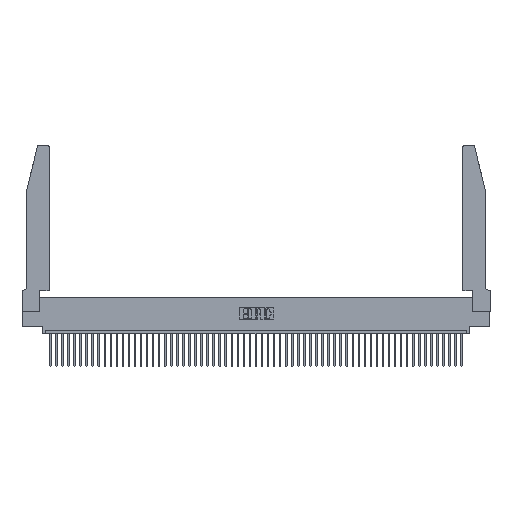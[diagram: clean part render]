
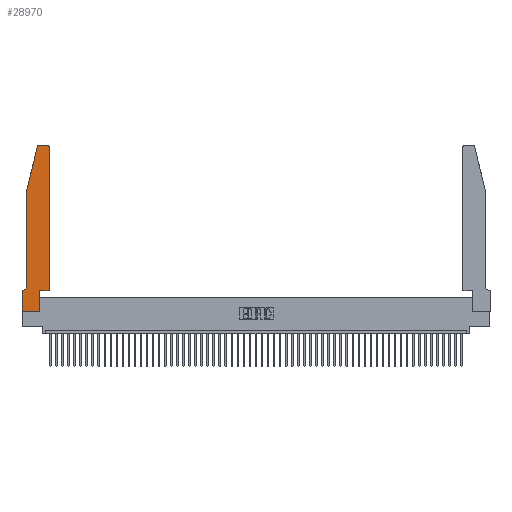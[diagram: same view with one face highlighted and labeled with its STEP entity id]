
A CAD part, top view. The second image highlights one B-rep face of the part: STEP entity #28970.
In plain terms, the highlighted planar face has unit normal (0, 0, 1).
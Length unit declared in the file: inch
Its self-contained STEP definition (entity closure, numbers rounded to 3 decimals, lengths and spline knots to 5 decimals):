
#1475 = DIRECTION ( 'NONE',  ( 1., 0., 0. ) ) ;
#1679 = CARTESIAN_POINT ( 'NONE',  ( 0.0055, 0.42, 0.37 ) ) ;
#3489 = ORIENTED_EDGE ( 'NONE', *, *, #41861, .T. ) ;
#3600 = VERTEX_POINT ( 'NONE', #26596 ) ;
#3605 = CARTESIAN_POINT ( 'NONE',  ( 0.284, 2.72, 0.37 ) ) ;
#3964 = CIRCLE ( 'NONE', #41250, 0.03 ) ;
#4069 = VECTOR ( 'NONE', #41590, 39.37008 ) ;
#4120 = CARTESIAN_POINT ( 'NONE',  ( 0.2865, 0.35, 0.37 ) ) ;
#4166 = VECTOR ( 'NONE', #1475, 39.37008 ) ;
#4811 = DIRECTION ( 'NONE',  ( 1., 0., 0. ) ) ;
#4860 = CARTESIAN_POINT ( 'NONE',  ( 0.284, 2.75, 0.37 ) ) ;
#5634 = DIRECTION ( 'NONE',  ( 0., 0., -1. ) ) ;
#5799 = ORIENTED_EDGE ( 'NONE', *, *, #6700, .T. ) ;
#5880 = CARTESIAN_POINT ( 'NONE',  ( 0.4205, 2.75, 0.37 ) ) ;
#5893 = VECTOR ( 'NONE', #17715, 39.37008 ) ;
#6623 = VECTOR ( 'NONE', #4811, 39.37008 ) ;
#6649 = DIRECTION ( 'NONE',  ( 0., 1., 0. ) ) ;
#6700 = EDGE_CURVE ( 'NONE', #46711, #46888, #7186, .T. ) ;
#7186 = LINE ( 'NONE', #13569, #5893 ) ;
#7447 = ORIENTED_EDGE ( 'NONE', *, *, #45981, .T. ) ;
#7721 = DIRECTION ( 'NONE',  ( 0., 0., 1. ) ) ;
#8319 = VECTOR ( 'NONE', #17550, 39.37008 ) ;
#8519 = LINE ( 'NONE', #19050, #6623 ) ;
#8619 = LINE ( 'NONE', #27113, #40102 ) ;
#9306 = CARTESIAN_POINT ( 'NONE',  ( 0.4505, 0.35, 0.37 ) ) ;
#10600 = EDGE_CURVE ( 'NONE', #15164, #21936, #8619, .T. ) ;
#10868 = CARTESIAN_POINT ( 'NONE',  ( 0., 0., 0.37 ) ) ;
#11533 = EDGE_CURVE ( 'NONE', #3600, #37272, #23302, .T. ) ;
#12237 = EDGE_CURVE ( 'NONE', #37272, #35717, #16134, .T. ) ;
#13504 = ORIENTED_EDGE ( 'NONE', *, *, #31787, .T. ) ;
#13569 = CARTESIAN_POINT ( 'NONE',  ( 0.0755, 2., 0.37 ) ) ;
#14154 = EDGE_CURVE ( 'NONE', #21936, #22428, #47812, .T. ) ;
#14614 = EDGE_CURVE ( 'NONE', #33912, #46142, #34206, .T. ) ;
#15164 = VERTEX_POINT ( 'NONE', #40572 ) ;
#15652 = AXIS2_PLACEMENT_3D ( 'NONE', #41416, #24895, #16969 ) ;
#16134 = LINE ( 'NONE', #10868, #46992 ) ;
#16969 = DIRECTION ( 'NONE',  ( 1., 0., 0. ) ) ;
#17550 = DIRECTION ( 'NONE',  ( 0., 1., 0. ) ) ;
#17715 = DIRECTION ( 'NONE',  ( 0., -1., 0. ) ) ;
#19050 = CARTESIAN_POINT ( 'NONE',  ( 0., 0., 0.37 ) ) ;
#19489 = CARTESIAN_POINT ( 'NONE',  ( 0.4505, 0.35, 0.37 ) ) ;
#19859 = CARTESIAN_POINT ( 'NONE',  ( 0.2605, 2.75, 0.37 ) ) ;
#21606 = LINE ( 'NONE', #19859, #44747 ) ;
#21936 = VERTEX_POINT ( 'NONE', #4120 ) ;
#22428 = VERTEX_POINT ( 'NONE', #19489 ) ;
#22996 = ORIENTED_EDGE ( 'NONE', *, *, #44598, .T. ) ;
#23302 = LINE ( 'NONE', #24395, #4069 ) ;
#23783 = CARTESIAN_POINT ( 'NONE',  ( 0.4205, 2.72, 0.37 ) ) ;
#24395 = CARTESIAN_POINT ( 'NONE',  ( 0.0755, 0.35, 0.37 ) ) ;
#24829 = DIRECTION ( 'NONE',  ( 0., -1., 0. ) ) ;
#24895 = DIRECTION ( 'NONE',  ( 0., 0., 1. ) ) ;
#25744 = ORIENTED_EDGE ( 'NONE', *, *, #10600, .T. ) ;
#26596 = CARTESIAN_POINT ( 'NONE',  ( 0.0055, 0.35, 0.37 ) ) ;
#26950 = VERTEX_POINT ( 'NONE', #47590 ) ;
#26964 = FACE_OUTER_BOUND ( 'NONE', #44069, .T. ) ;
#27113 = CARTESIAN_POINT ( 'NONE',  ( 0.2865, 0.35, 0.37 ) ) ;
#27609 = DIRECTION ( 'NONE',  ( -1., 0., 0. ) ) ;
#28302 = DIRECTION ( 'NONE',  ( 0., 0., 1. ) ) ;
#28970 = ADVANCED_FACE ( 'NONE', ( #26964 ), #49310, .T. ) ;
#31787 = EDGE_CURVE ( 'NONE', #46888, #3600, #46589, .T. ) ;
#31884 = DIRECTION ( 'NONE',  ( 1., 0., 0. ) ) ;
#33912 = VERTEX_POINT ( 'NONE', #33946 ) ;
#33946 = CARTESIAN_POINT ( 'NONE',  ( 0.4505, 2.72, 0.37 ) ) ;
#34206 = CIRCLE ( 'NONE', #36188, 0.03 ) ;
#34320 = AXIS2_PLACEMENT_3D ( 'NONE', #1679, #5634, #38463 ) ;
#35717 = VERTEX_POINT ( 'NONE', #46463 ) ;
#36188 = AXIS2_PLACEMENT_3D ( 'NONE', #23783, #28302, #31884 ) ;
#36679 = CARTESIAN_POINT ( 'NONE',  ( 0.0755, 0.42, 0.37 ) ) ;
#36992 = CARTESIAN_POINT ( 'NONE',  ( 0., 0.35, 0.37 ) ) ;
#37272 = VERTEX_POINT ( 'NONE', #36992 ) ;
#38132 = CARTESIAN_POINT ( 'NONE',  ( 0.0755, 2., 0.37 ) ) ;
#38463 = DIRECTION ( 'NONE',  ( -1., 0., 0. ) ) ;
#40102 = VECTOR ( 'NONE', #6649, 39.37008 ) ;
#40572 = CARTESIAN_POINT ( 'NONE',  ( 0.2865, 0., 0.37 ) ) ;
#40919 = ORIENTED_EDGE ( 'NONE', *, *, #11533, .T. ) ;
#41250 = AXIS2_PLACEMENT_3D ( 'NONE', #3605, #7721, #48647 ) ;
#41330 = VECTOR ( 'NONE', #42250, 39.37008 ) ;
#41416 = CARTESIAN_POINT ( 'NONE',  ( 0., 0.35, 0.37 ) ) ;
#41590 = DIRECTION ( 'NONE',  ( -1., 0., 0. ) ) ;
#41861 = EDGE_CURVE ( 'NONE', #46142, #44980, #21606, .T. ) ;
#42250 = DIRECTION ( 'NONE',  ( -0.239, -0.971, 0. ) ) ;
#43334 = ORIENTED_EDGE ( 'NONE', *, *, #49544, .T. ) ;
#43576 = EDGE_CURVE ( 'NONE', #35717, #15164, #8519, .T. ) ;
#44069 = EDGE_LOOP ( 'NONE', ( #3489, #22996, #43334, #5799, #13504, #40919, #49337, #52206, #25744, #52599, #7447, #52835 ) ) ;
#44598 = EDGE_CURVE ( 'NONE', #44980, #26950, #3964, .T. ) ;
#44747 = VECTOR ( 'NONE', #27609, 39.37008 ) ;
#44980 = VERTEX_POINT ( 'NONE', #4860 ) ;
#45600 = CARTESIAN_POINT ( 'NONE',  ( 0.4505, 0.35, 0.37 ) ) ;
#45981 = EDGE_CURVE ( 'NONE', #22428, #33912, #50068, .T. ) ;
#46142 = VERTEX_POINT ( 'NONE', #5880 ) ;
#46463 = CARTESIAN_POINT ( 'NONE',  ( 0., 0., 0.37 ) ) ;
#46589 = CIRCLE ( 'NONE', #34320, 0.07 ) ;
#46711 = VERTEX_POINT ( 'NONE', #47097 ) ;
#46888 = VERTEX_POINT ( 'NONE', #36679 ) ;
#46992 = VECTOR ( 'NONE', #24829, 39.37008 ) ;
#47097 = CARTESIAN_POINT ( 'NONE',  ( 0.0755, 2., 0.37 ) ) ;
#47590 = CARTESIAN_POINT ( 'NONE',  ( 0.25487, 2.72718, 0.37 ) ) ;
#47812 = LINE ( 'NONE', #9306, #4166 ) ;
#48647 = DIRECTION ( 'NONE',  ( 1., 0., 0. ) ) ;
#49310 = PLANE ( 'NONE',  #15652 ) ;
#49337 = ORIENTED_EDGE ( 'NONE', *, *, #12237, .T. ) ;
#49544 = EDGE_CURVE ( 'NONE', #26950, #46711, #50291, .T. ) ;
#50068 = LINE ( 'NONE', #45600, #8319 ) ;
#50291 = LINE ( 'NONE', #38132, #41330 ) ;
#52206 = ORIENTED_EDGE ( 'NONE', *, *, #43576, .T. ) ;
#52599 = ORIENTED_EDGE ( 'NONE', *, *, #14154, .T. ) ;
#52835 = ORIENTED_EDGE ( 'NONE', *, *, #14614, .T. ) ;
